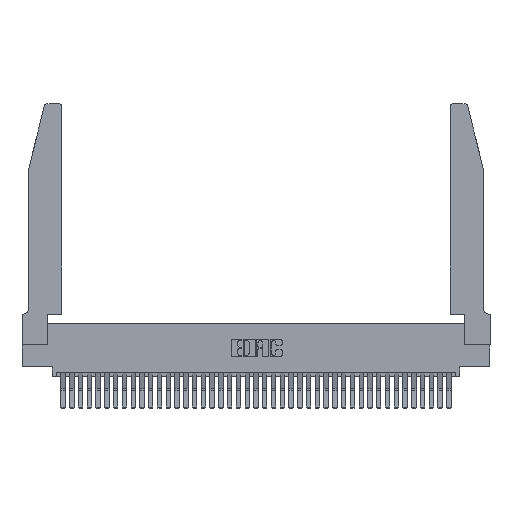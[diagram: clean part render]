
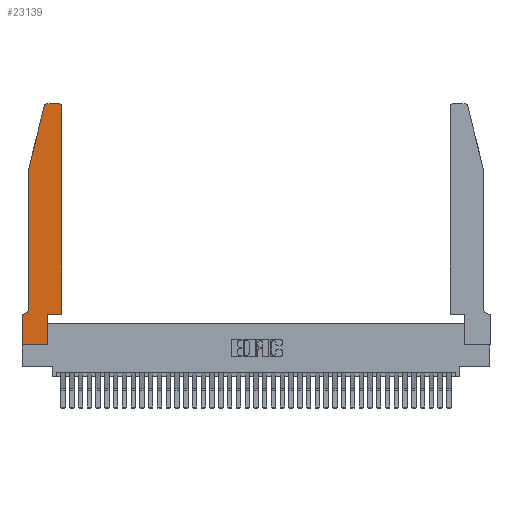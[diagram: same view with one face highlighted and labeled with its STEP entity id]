
A CAD part, top view. The second image highlights one B-rep face of the part: STEP entity #23139.
In plain terms, the highlighted planar face has unit normal (0, 0, 1).
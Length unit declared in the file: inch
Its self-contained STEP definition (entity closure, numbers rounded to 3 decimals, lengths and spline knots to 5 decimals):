
#277 = VERTEX_POINT ( 'NONE', #29733 ) ;
#518 = AXIS2_PLACEMENT_3D ( 'NONE', #39055, #5364, #5743 ) ;
#755 = CARTESIAN_POINT ( 'NONE',  ( 0.4505, 2.72, 0.37 ) ) ;
#1105 = CARTESIAN_POINT ( 'NONE',  ( 0.2865, 0.35, 0.37 ) ) ;
#1323 = ORIENTED_EDGE ( 'NONE', *, *, #31873, .T. ) ;
#2622 = CARTESIAN_POINT ( 'NONE',  ( 0., 0.35, 0.37 ) ) ;
#2820 = VECTOR ( 'NONE', #15149, 39.37008 ) ;
#3190 = CIRCLE ( 'NONE', #16865, 0.07 ) ;
#3355 = CARTESIAN_POINT ( 'NONE',  ( 0.0055, 0.35, 0.37 ) ) ;
#3475 = ORIENTED_EDGE ( 'NONE', *, *, #25334, .T. ) ;
#4468 = VECTOR ( 'NONE', #18016, 39.37008 ) ;
#5364 = DIRECTION ( 'NONE',  ( 0., 0., 1. ) ) ;
#5743 = DIRECTION ( 'NONE',  ( 1., 0., 0. ) ) ;
#5792 = VERTEX_POINT ( 'NONE', #2622 ) ;
#6478 = VERTEX_POINT ( 'NONE', #35086 ) ;
#6992 = CARTESIAN_POINT ( 'NONE',  ( 0.4205, 2.72, 0.37 ) ) ;
#7123 = VERTEX_POINT ( 'NONE', #3355 ) ;
#7464 = CARTESIAN_POINT ( 'NONE',  ( 0.4205, 2.75, 0.37 ) ) ;
#7622 = LINE ( 'NONE', #24388, #2820 ) ;
#8689 = AXIS2_PLACEMENT_3D ( 'NONE', #6992, #26737, #27012 ) ;
#9138 = FACE_OUTER_BOUND ( 'NONE', #38466, .T. ) ;
#9687 = VERTEX_POINT ( 'NONE', #16794 ) ;
#10191 = ORIENTED_EDGE ( 'NONE', *, *, #17546, .T. ) ;
#11899 = ORIENTED_EDGE ( 'NONE', *, *, #36692, .T. ) ;
#12781 = CARTESIAN_POINT ( 'NONE',  ( 0.0055, 0.42, 0.37 ) ) ;
#12878 = DIRECTION ( 'NONE',  ( 1., 0., 0. ) ) ;
#13488 = ORIENTED_EDGE ( 'NONE', *, *, #36257, .T. ) ;
#13513 = VECTOR ( 'NONE', #22660, 39.37008 ) ;
#14313 = CIRCLE ( 'NONE', #8689, 0.03 ) ;
#14473 = EDGE_CURVE ( 'NONE', #6478, #26480, #16485, .T. ) ;
#14611 = VECTOR ( 'NONE', #33320, 39.37008 ) ;
#14838 = VECTOR ( 'NONE', #15714, 39.37008 ) ;
#14893 = EDGE_CURVE ( 'NONE', #26480, #21426, #33821, .T. ) ;
#15022 = AXIS2_PLACEMENT_3D ( 'NONE', #19252, #19114, #12878 ) ;
#15149 = DIRECTION ( 'NONE',  ( -1., 0., 0. ) ) ;
#15580 = CARTESIAN_POINT ( 'NONE',  ( 0.4505, 0.35, 0.37 ) ) ;
#15714 = DIRECTION ( 'NONE',  ( 0., 1., 0. ) ) ;
#15867 = DIRECTION ( 'NONE',  ( 0., 0., -1. ) ) ;
#16216 = ORIENTED_EDGE ( 'NONE', *, *, #14893, .T. ) ;
#16485 = LINE ( 'NONE', #38801, #4468 ) ;
#16794 = CARTESIAN_POINT ( 'NONE',  ( 0.4505, 0.35, 0.37 ) ) ;
#16865 = AXIS2_PLACEMENT_3D ( 'NONE', #12781, #15867, #25213 ) ;
#17546 = EDGE_CURVE ( 'NONE', #21828, #25611, #14313, .T. ) ;
#18016 = DIRECTION ( 'NONE',  ( 1., 0., 0. ) ) ;
#18042 = LINE ( 'NONE', #18923, #37785 ) ;
#18590 = VECTOR ( 'NONE', #33481, 39.37008 ) ;
#18923 = CARTESIAN_POINT ( 'NONE',  ( 0.0755, 0.35, 0.37 ) ) ;
#19114 = DIRECTION ( 'NONE',  ( 0., 0., 1. ) ) ;
#19182 = DIRECTION ( 'NONE',  ( -1., 0., 0. ) ) ;
#19252 = CARTESIAN_POINT ( 'NONE',  ( 0., 0.35, 0.37 ) ) ;
#19572 = EDGE_CURVE ( 'NONE', #7123, #5792, #18042, .T. ) ;
#20532 = CARTESIAN_POINT ( 'NONE',  ( 0.0755, 2., 0.37 ) ) ;
#21082 = ORIENTED_EDGE ( 'NONE', *, *, #35502, .T. ) ;
#21426 = VERTEX_POINT ( 'NONE', #28958 ) ;
#21548 = CARTESIAN_POINT ( 'NONE',  ( 0.4505, 0.35, 0.37 ) ) ;
#21559 = ORIENTED_EDGE ( 'NONE', *, *, #19572, .T. ) ;
#21828 = VERTEX_POINT ( 'NONE', #755 ) ;
#22660 = DIRECTION ( 'NONE',  ( 0., 1., 0. ) ) ;
#23097 = LINE ( 'NONE', #15580, #14838 ) ;
#23139 = ADVANCED_FACE ( 'NONE', ( #9138 ), #31096, .T. ) ;
#23913 = ORIENTED_EDGE ( 'NONE', *, *, #24863, .T. ) ;
#24388 = CARTESIAN_POINT ( 'NONE',  ( 0.2605, 2.75, 0.37 ) ) ;
#24863 = EDGE_CURVE ( 'NONE', #9687, #21828, #23097, .T. ) ;
#25213 = DIRECTION ( 'NONE',  ( -1., 0., 0. ) ) ;
#25334 = EDGE_CURVE ( 'NONE', #25611, #36938, #7622, .T. ) ;
#25611 = VERTEX_POINT ( 'NONE', #7464 ) ;
#25661 = ORIENTED_EDGE ( 'NONE', *, *, #37527, .T. ) ;
#26290 = VERTEX_POINT ( 'NONE', #29434 ) ;
#26375 = ORIENTED_EDGE ( 'NONE', *, *, #38936, .T. ) ;
#26480 = VERTEX_POINT ( 'NONE', #35345 ) ;
#26737 = DIRECTION ( 'NONE',  ( 0., 0., 1. ) ) ;
#26754 = LINE ( 'NONE', #21548, #35888 ) ;
#26826 = VERTEX_POINT ( 'NONE', #33179 ) ;
#27012 = DIRECTION ( 'NONE',  ( 1., 0., 0. ) ) ;
#28958 = CARTESIAN_POINT ( 'NONE',  ( 0.2865, 0.35, 0.37 ) ) ;
#29434 = CARTESIAN_POINT ( 'NONE',  ( 0.0755, 2., 0.37 ) ) ;
#29733 = CARTESIAN_POINT ( 'NONE',  ( 0.0755, 0.42, 0.37 ) ) ;
#31096 = PLANE ( 'NONE',  #15022 ) ;
#31873 = EDGE_CURVE ( 'NONE', #36938, #26826, #35083, .T. ) ;
#32605 = DIRECTION ( 'NONE',  ( -0.239, -0.971, 0. ) ) ;
#33054 = CARTESIAN_POINT ( 'NONE',  ( 0.0755, 2., 0.37 ) ) ;
#33179 = CARTESIAN_POINT ( 'NONE',  ( 0.25487, 2.72718, 0.37 ) ) ;
#33320 = DIRECTION ( 'NONE',  ( 0., -1., 0. ) ) ;
#33481 = DIRECTION ( 'NONE',  ( 0., -1., 0. ) ) ;
#33821 = LINE ( 'NONE', #1105, #13513 ) ;
#34412 = ORIENTED_EDGE ( 'NONE', *, *, #14473, .T. ) ;
#35083 = CIRCLE ( 'NONE', #518, 0.03 ) ;
#35086 = CARTESIAN_POINT ( 'NONE',  ( 0., 0., 0.37 ) ) ;
#35233 = LINE ( 'NONE', #20532, #39114 ) ;
#35345 = CARTESIAN_POINT ( 'NONE',  ( 0.2865, 0., 0.37 ) ) ;
#35502 = EDGE_CURVE ( 'NONE', #5792, #6478, #37360, .T. ) ;
#35888 = VECTOR ( 'NONE', #36891, 39.37008 ) ;
#36257 = EDGE_CURVE ( 'NONE', #277, #7123, #3190, .T. ) ;
#36692 = EDGE_CURVE ( 'NONE', #21426, #9687, #26754, .T. ) ;
#36891 = DIRECTION ( 'NONE',  ( 1., 0., 0. ) ) ;
#36938 = VERTEX_POINT ( 'NONE', #38231 ) ;
#37360 = LINE ( 'NONE', #39829, #18590 ) ;
#37527 = EDGE_CURVE ( 'NONE', #26290, #277, #39674, .T. ) ;
#37785 = VECTOR ( 'NONE', #19182, 39.37008 ) ;
#38231 = CARTESIAN_POINT ( 'NONE',  ( 0.284, 2.75, 0.37 ) ) ;
#38466 = EDGE_LOOP ( 'NONE', ( #3475, #1323, #26375, #25661, #13488, #21559, #21082, #34412, #16216, #11899, #23913, #10191 ) ) ;
#38801 = CARTESIAN_POINT ( 'NONE',  ( 0., 0., 0.37 ) ) ;
#38936 = EDGE_CURVE ( 'NONE', #26826, #26290, #35233, .T. ) ;
#39055 = CARTESIAN_POINT ( 'NONE',  ( 0.284, 2.72, 0.37 ) ) ;
#39114 = VECTOR ( 'NONE', #32605, 39.37008 ) ;
#39674 = LINE ( 'NONE', #33054, #14611 ) ;
#39829 = CARTESIAN_POINT ( 'NONE',  ( 0., 0., 0.37 ) ) ;
